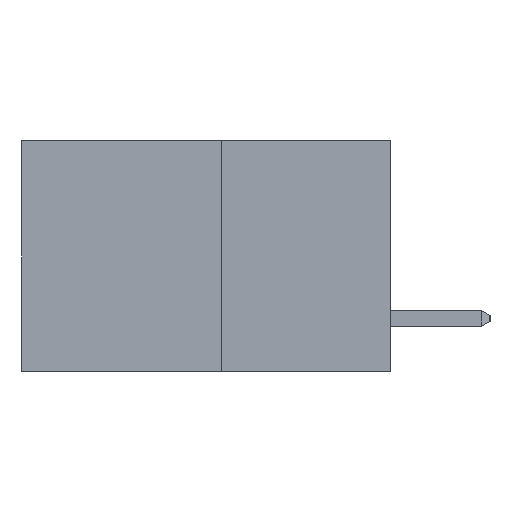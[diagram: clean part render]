
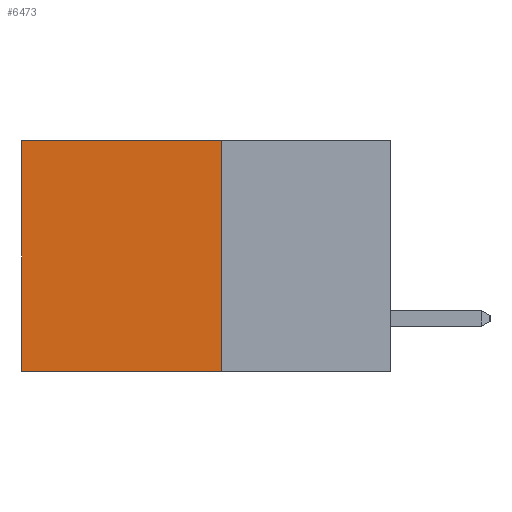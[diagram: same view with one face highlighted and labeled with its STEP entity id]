
A CAD part, left-side view. The second image highlights one B-rep face of the part: STEP entity #6473.
In plain terms, the highlighted planar face has unit normal (-1, 0, 0).
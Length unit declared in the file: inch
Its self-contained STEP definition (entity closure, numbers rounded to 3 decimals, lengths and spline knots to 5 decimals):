
#225 = EDGE_CURVE ( 'NONE', #14540, #2721, #18078, .T. ) ;
#667 = LINE ( 'NONE', #2029, #12348 ) ;
#849 = VERTEX_POINT ( 'NONE', #14748 ) ;
#1337 = EDGE_CURVE ( 'NONE', #6397, #2721, #18269, .T. ) ;
#2029 = CARTESIAN_POINT ( 'NONE',  ( 0.277, 0.27, -0.37 ) ) ;
#2308 = VECTOR ( 'NONE', #4433, 39.37008 ) ;
#2721 = VERTEX_POINT ( 'NONE', #13217 ) ;
#3544 = CARTESIAN_POINT ( 'NONE',  ( 0.277, 0.27, -0.37 ) ) ;
#3755 = ORIENTED_EDGE ( 'NONE', *, *, #8863, .F. ) ;
#4433 = DIRECTION ( 'NONE',  ( 0., 0., -1. ) ) ;
#4939 = EDGE_CURVE ( 'NONE', #849, #6397, #11368, .T. ) ;
#5581 = CARTESIAN_POINT ( 'NONE',  ( 0.277, 0.59, -0.37 ) ) ;
#6397 = VERTEX_POINT ( 'NONE', #14926 ) ;
#6473 = ADVANCED_FACE ( 'NONE', ( #18910 ), #13797, .F. ) ;
#7778 = ORIENTED_EDGE ( 'NONE', *, *, #4939, .T. ) ;
#8452 = DIRECTION ( 'NONE',  ( 0., 1., 0. ) ) ;
#8699 = CARTESIAN_POINT ( 'NONE',  ( 0.277, 0.27, 0. ) ) ;
#8863 = EDGE_CURVE ( 'NONE', #849, #14540, #667, .T. ) ;
#9736 = DIRECTION ( 'NONE',  ( 0., 0., -1. ) ) ;
#10862 = ORIENTED_EDGE ( 'NONE', *, *, #1337, .T. ) ;
#11368 = LINE ( 'NONE', #8699, #15250 ) ;
#12348 = VECTOR ( 'NONE', #9736, 39.37008 ) ;
#13217 = CARTESIAN_POINT ( 'NONE',  ( 0.277, 0.59, -0.37 ) ) ;
#13593 = AXIS2_PLACEMENT_3D ( 'NONE', #13792, #13770, #13752 ) ;
#13752 = DIRECTION ( 'NONE',  ( 0., 0., -1. ) ) ;
#13770 = DIRECTION ( 'NONE',  ( 1., 0., 0. ) ) ;
#13792 = CARTESIAN_POINT ( 'NONE',  ( 0.277, 0.27, -0.37 ) ) ;
#13797 = PLANE ( 'NONE',  #13593 ) ;
#14540 = VERTEX_POINT ( 'NONE', #3544 ) ;
#14748 = CARTESIAN_POINT ( 'NONE',  ( 0.277, 0.27, 0. ) ) ;
#14926 = CARTESIAN_POINT ( 'NONE',  ( 0.277, 0.59, 0. ) ) ;
#15250 = VECTOR ( 'NONE', #8452, 39.37008 ) ;
#17171 = DIRECTION ( 'NONE',  ( 0., 1., 0. ) ) ;
#17618 = VECTOR ( 'NONE', #17171, 39.37008 ) ;
#18078 = LINE ( 'NONE', #19289, #17618 ) ;
#18269 = LINE ( 'NONE', #5581, #2308 ) ;
#18699 = EDGE_LOOP ( 'NONE', ( #10862, #19137, #3755, #7778 ) ) ;
#18910 = FACE_OUTER_BOUND ( 'NONE', #18699, .T. ) ;
#19137 = ORIENTED_EDGE ( 'NONE', *, *, #225, .F. ) ;
#19289 = CARTESIAN_POINT ( 'NONE',  ( 0.277, 0.27, -0.37 ) ) ;
